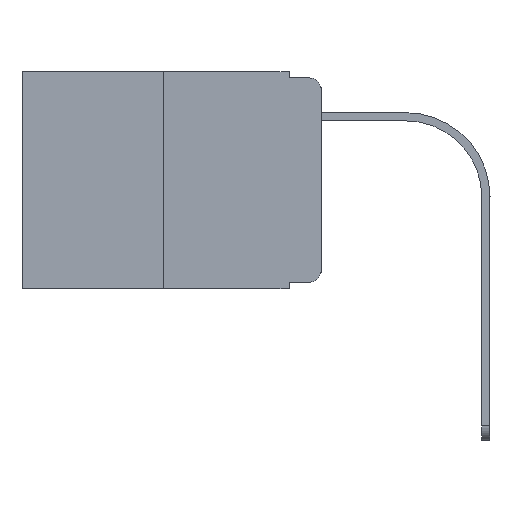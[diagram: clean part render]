
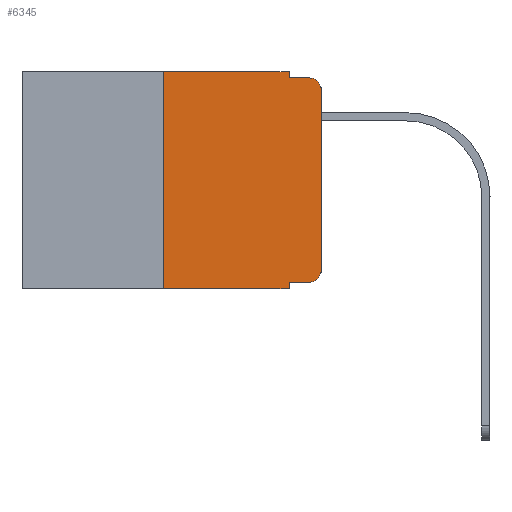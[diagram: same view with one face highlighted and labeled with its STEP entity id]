
A CAD part, left-side view. The second image highlights one B-rep face of the part: STEP entity #6345.
In plain terms, the highlighted planar face has unit normal (-1, 0, 0).
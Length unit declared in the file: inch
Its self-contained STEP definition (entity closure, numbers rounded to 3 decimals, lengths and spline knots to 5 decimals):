
#203 = CARTESIAN_POINT ( 'NONE',  ( 0., 0.051, -0.01 ) ) ;
#296 = AXIS2_PLACEMENT_3D ( 'NONE', #1873, #7537, #432 ) ;
#340 = LINE ( 'NONE', #203, #3113 ) ;
#386 = ORIENTED_EDGE ( 'NONE', *, *, #7460, .T. ) ;
#388 = ORIENTED_EDGE ( 'NONE', *, *, #2225, .F. ) ;
#432 = DIRECTION ( 'NONE',  ( 0., 0., -1. ) ) ;
#457 = DIRECTION ( 'NONE',  ( 0., -1., 0. ) ) ;
#476 = EDGE_CURVE ( 'NONE', #9469, #5478, #2513, .T. ) ;
#606 = EDGE_CURVE ( 'NONE', #9447, #901, #340, .T. ) ;
#697 = CARTESIAN_POINT ( 'NONE',  ( 0., 0.051, 0. ) ) ;
#800 = VECTOR ( 'NONE', #9521, 39.37008 ) ;
#805 = CARTESIAN_POINT ( 'NONE',  ( 0., 0.473, 0. ) ) ;
#847 = VECTOR ( 'NONE', #10259, 39.37008 ) ;
#859 = CARTESIAN_POINT ( 'NONE',  ( 0., 0.02, -0.01 ) ) ;
#901 = VERTEX_POINT ( 'NONE', #859 ) ;
#933 = DIRECTION ( 'NONE',  ( 0., 0., -1. ) ) ;
#1008 = LINE ( 'NONE', #8144, #1432 ) ;
#1011 = VECTOR ( 'NONE', #457, 39.37008 ) ;
#1385 = VERTEX_POINT ( 'NONE', #1684 ) ;
#1432 = VECTOR ( 'NONE', #7400, 39.37008 ) ;
#1479 = DIRECTION ( 'NONE',  ( 1., 0., 0. ) ) ;
#1581 = VERTEX_POINT ( 'NONE', #8996 ) ;
#1598 = EDGE_LOOP ( 'NONE', ( #5995, #386, #9292, #8791, #388, #3709, #5965, #6958, #5610, #6929 ) ) ;
#1684 = CARTESIAN_POINT ( 'NONE',  ( 0., 0., -0.03 ) ) ;
#1793 = CARTESIAN_POINT ( 'NONE',  ( 0., 0.25, -0.343 ) ) ;
#1873 = CARTESIAN_POINT ( 'NONE',  ( 0., 0.02, -0.03 ) ) ;
#1906 = VERTEX_POINT ( 'NONE', #4049 ) ;
#2225 = EDGE_CURVE ( 'NONE', #5478, #3603, #5780, .T. ) ;
#2304 = CIRCLE ( 'NONE', #296, 0.02 ) ;
#2453 = EDGE_CURVE ( 'NONE', #6448, #1906, #6286, .T. ) ;
#2502 = VECTOR ( 'NONE', #5226, 39.37008 ) ;
#2513 = LINE ( 'NONE', #8918, #9046 ) ;
#2734 = CIRCLE ( 'NONE', #9638, 0.02 ) ;
#2921 = EDGE_CURVE ( 'NONE', #3603, #9447, #5423, .T. ) ;
#2971 = VERTEX_POINT ( 'NONE', #7278 ) ;
#3078 = LINE ( 'NONE', #697, #847 ) ;
#3113 = VECTOR ( 'NONE', #7592, 39.37008 ) ;
#3603 = VERTEX_POINT ( 'NONE', #8236 ) ;
#3709 = ORIENTED_EDGE ( 'NONE', *, *, #476, .F. ) ;
#3864 = PLANE ( 'NONE',  #10290 ) ;
#4049 = CARTESIAN_POINT ( 'NONE',  ( 0., 0.02, -0.333 ) ) ;
#4519 = LINE ( 'NONE', #6164, #1011 ) ;
#5065 = CARTESIAN_POINT ( 'NONE',  ( 0., 0.051, -0.01 ) ) ;
#5226 = DIRECTION ( 'NONE',  ( 0., 0., -1. ) ) ;
#5338 = CARTESIAN_POINT ( 'NONE',  ( 0., 0.473, 0. ) ) ;
#5374 = CARTESIAN_POINT ( 'NONE',  ( 0., 0.051, 0. ) ) ;
#5423 = LINE ( 'NONE', #5374, #2502 ) ;
#5438 = EDGE_CURVE ( 'NONE', #9469, #1581, #4519, .T. ) ;
#5478 = VERTEX_POINT ( 'NONE', #7808 ) ;
#5572 = DIRECTION ( 'NONE',  ( 0., 0., 1. ) ) ;
#5610 = ORIENTED_EDGE ( 'NONE', *, *, #2453, .T. ) ;
#5780 = LINE ( 'NONE', #805, #6704 ) ;
#5965 = ORIENTED_EDGE ( 'NONE', *, *, #5438, .T. ) ;
#5995 = ORIENTED_EDGE ( 'NONE', *, *, #9507, .T. ) ;
#6164 = CARTESIAN_POINT ( 'NONE',  ( 0., 0.473, -0.343 ) ) ;
#6242 = CARTESIAN_POINT ( 'NONE',  ( 0., 0.051, -0.333 ) ) ;
#6286 = LINE ( 'NONE', #10097, #800 ) ;
#6339 = DIRECTION ( 'NONE',  ( 0., 0., -1. ) ) ;
#6345 = ADVANCED_FACE ( 'NONE', ( #9373 ), #3864, .F. ) ;
#6445 = EDGE_CURVE ( 'NONE', #6448, #1581, #3078, .T. ) ;
#6448 = VERTEX_POINT ( 'NONE', #6242 ) ;
#6704 = VECTOR ( 'NONE', #8651, 39.37008 ) ;
#6929 = ORIENTED_EDGE ( 'NONE', *, *, #6998, .T. ) ;
#6958 = ORIENTED_EDGE ( 'NONE', *, *, #6445, .F. ) ;
#6998 = EDGE_CURVE ( 'NONE', #1906, #2971, #2734, .T. ) ;
#7278 = CARTESIAN_POINT ( 'NONE',  ( 0., 0., -0.313 ) ) ;
#7400 = DIRECTION ( 'NONE',  ( 0., 0., 1. ) ) ;
#7460 = EDGE_CURVE ( 'NONE', #1385, #901, #2304, .T. ) ;
#7537 = DIRECTION ( 'NONE',  ( -1., 0., 0. ) ) ;
#7592 = DIRECTION ( 'NONE',  ( 0., -1., 0. ) ) ;
#7808 = CARTESIAN_POINT ( 'NONE',  ( 0., 0.25, 0. ) ) ;
#8144 = CARTESIAN_POINT ( 'NONE',  ( 0., 0., 0. ) ) ;
#8182 = DIRECTION ( 'NONE',  ( -1., 0., 0. ) ) ;
#8236 = CARTESIAN_POINT ( 'NONE',  ( 0., 0.051, 0. ) ) ;
#8651 = DIRECTION ( 'NONE',  ( 0., -1., 0. ) ) ;
#8791 = ORIENTED_EDGE ( 'NONE', *, *, #2921, .F. ) ;
#8918 = CARTESIAN_POINT ( 'NONE',  ( 0., 0.25, 0. ) ) ;
#8996 = CARTESIAN_POINT ( 'NONE',  ( 0., 0.051, -0.343 ) ) ;
#9046 = VECTOR ( 'NONE', #5572, 39.37008 ) ;
#9292 = ORIENTED_EDGE ( 'NONE', *, *, #606, .F. ) ;
#9373 = FACE_OUTER_BOUND ( 'NONE', #1598, .T. ) ;
#9447 = VERTEX_POINT ( 'NONE', #5065 ) ;
#9469 = VERTEX_POINT ( 'NONE', #1793 ) ;
#9507 = EDGE_CURVE ( 'NONE', #2971, #1385, #1008, .T. ) ;
#9521 = DIRECTION ( 'NONE',  ( 0., -1., 0. ) ) ;
#9638 = AXIS2_PLACEMENT_3D ( 'NONE', #9817, #8182, #933 ) ;
#9817 = CARTESIAN_POINT ( 'NONE',  ( 0., 0.02, -0.313 ) ) ;
#10097 = CARTESIAN_POINT ( 'NONE',  ( 0., 0.051, -0.333 ) ) ;
#10259 = DIRECTION ( 'NONE',  ( 0., 0., -1. ) ) ;
#10290 = AXIS2_PLACEMENT_3D ( 'NONE', #5338, #1479, #6339 ) ;
